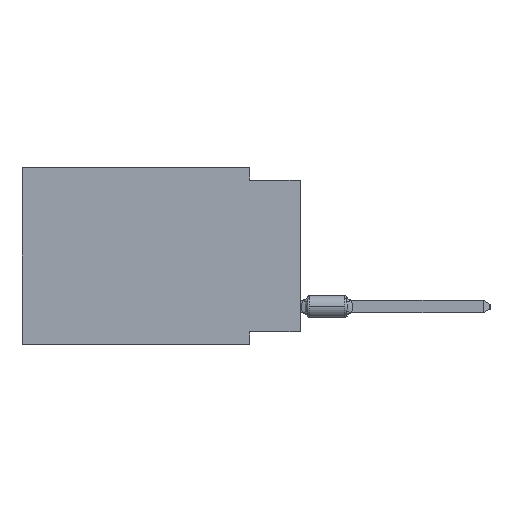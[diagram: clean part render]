
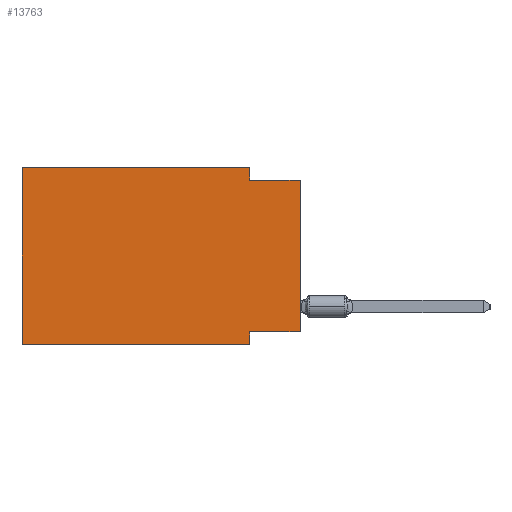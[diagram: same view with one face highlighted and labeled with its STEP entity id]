
A CAD part, left-side view. The second image highlights one B-rep face of the part: STEP entity #13763.
In plain terms, the highlighted planar face has unit normal (-1, 0, 0).
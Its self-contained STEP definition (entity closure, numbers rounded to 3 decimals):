
#1804 = CARTESIAN_POINT ( 'NONE',  ( 0., 13.97, 0. ) ) ;
#2532 = VERTEX_POINT ( 'NONE', #74510 ) ;
#4743 = VERTEX_POINT ( 'NONE', #37701 ) ;
#6497 = CARTESIAN_POINT ( 'NONE',  ( 0., 2.54, -8.255 ) ) ;
#6792 = DIRECTION ( 'NONE',  ( 0., -1., 0. ) ) ;
#8839 = DIRECTION ( 'NONE',  ( 0., -1., 0. ) ) ;
#11385 = EDGE_CURVE ( 'NONE', #55687, #71116, #38033, .T. ) ;
#11676 = VERTEX_POINT ( 'NONE', #31573 ) ;
#13763 = ADVANCED_FACE ( 'NONE', ( #26421 ), #49687, .F. ) ;
#14637 = VERTEX_POINT ( 'NONE', #60135 ) ;
#14918 = VECTOR ( 'NONE', #97933, 1000. ) ;
#18485 = CARTESIAN_POINT ( 'NONE',  ( 0., 13.97, 0. ) ) ;
#21671 = VERTEX_POINT ( 'NONE', #64441 ) ;
#23043 = LINE ( 'NONE', #67661, #14918 ) ;
#23168 = DIRECTION ( 'NONE',  ( 0., 0., -1. ) ) ;
#23503 = EDGE_CURVE ( 'NONE', #11676, #72707, #46404, .T. ) ;
#25033 = EDGE_CURVE ( 'NONE', #2532, #4743, #72565, .T. ) ;
#25195 = ORIENTED_EDGE ( 'NONE', *, *, #33677, .F. ) ;
#26421 = FACE_OUTER_BOUND ( 'NONE', #36761, .T. ) ;
#28302 = LINE ( 'NONE', #72433, #88564 ) ;
#31462 = ORIENTED_EDGE ( 'NONE', *, *, #58525, .T. ) ;
#31573 = CARTESIAN_POINT ( 'NONE',  ( 0., 13.97, 0. ) ) ;
#32923 = CARTESIAN_POINT ( 'NONE',  ( 0., 2.54, 0. ) ) ;
#33677 = EDGE_CURVE ( 'NONE', #2532, #55687, #85580, .T. ) ;
#34881 = CARTESIAN_POINT ( 'NONE',  ( 0., 0., 0. ) ) ;
#35316 = VECTOR ( 'NONE', #8839, 1000. ) ;
#36761 = EDGE_LOOP ( 'NONE', ( #65726, #79341, #88695, #41415, #40540, #31462, #63442, #25195 ) ) ;
#37701 = CARTESIAN_POINT ( 'NONE',  ( 0., 0., -0.635 ) ) ;
#38033 = LINE ( 'NONE', #60830, #38064 ) ;
#38064 = VECTOR ( 'NONE', #23168, 1000. ) ;
#40540 = ORIENTED_EDGE ( 'NONE', *, *, #73470, .F. ) ;
#40972 = VECTOR ( 'NONE', #6792, 1000. ) ;
#41415 = ORIENTED_EDGE ( 'NONE', *, *, #23503, .F. ) ;
#46404 = LINE ( 'NONE', #53337, #40972 ) ;
#46496 = CARTESIAN_POINT ( 'NONE',  ( 0., 13.97, -8.89 ) ) ;
#48286 = DIRECTION ( 'NONE',  ( 0., 0., 1. ) ) ;
#49687 = PLANE ( 'NONE',  #96887 ) ;
#52313 = EDGE_CURVE ( 'NONE', #72707, #14637, #28302, .T. ) ;
#53337 = CARTESIAN_POINT ( 'NONE',  ( 0., 13.97, 0. ) ) ;
#54364 = DIRECTION ( 'NONE',  ( 0., 0., 1. ) ) ;
#54808 = DIRECTION ( 'NONE',  ( 0., 1., 0. ) ) ;
#55396 = LINE ( 'NONE', #46496, #35316 ) ;
#55687 = VERTEX_POINT ( 'NONE', #6497 ) ;
#56162 = DIRECTION ( 'NONE',  ( 0., 0., -1. ) ) ;
#58525 = EDGE_CURVE ( 'NONE', #21671, #71116, #55396, .T. ) ;
#60135 = CARTESIAN_POINT ( 'NONE',  ( 0., 2.54, -0.635 ) ) ;
#60830 = CARTESIAN_POINT ( 'NONE',  ( 0., 2.54, -8.89 ) ) ;
#61460 = EDGE_CURVE ( 'NONE', #14637, #4743, #23043, .T. ) ;
#63442 = ORIENTED_EDGE ( 'NONE', *, *, #11385, .F. ) ;
#64441 = CARTESIAN_POINT ( 'NONE',  ( 0., 13.97, -8.89 ) ) ;
#64725 = VECTOR ( 'NONE', #54364, 1000. ) ;
#64823 = VECTOR ( 'NONE', #54808, 1000. ) ;
#65726 = ORIENTED_EDGE ( 'NONE', *, *, #25033, .T. ) ;
#67661 = CARTESIAN_POINT ( 'NONE',  ( 0., 0., -0.635 ) ) ;
#71116 = VERTEX_POINT ( 'NONE', #94997 ) ;
#72433 = CARTESIAN_POINT ( 'NONE',  ( 0., 2.54, 0. ) ) ;
#72565 = LINE ( 'NONE', #34881, #81069 ) ;
#72707 = VERTEX_POINT ( 'NONE', #32923 ) ;
#73470 = EDGE_CURVE ( 'NONE', #21671, #11676, #77192, .T. ) ;
#74510 = CARTESIAN_POINT ( 'NONE',  ( 0., 0., -8.255 ) ) ;
#77192 = LINE ( 'NONE', #1804, #64725 ) ;
#79341 = ORIENTED_EDGE ( 'NONE', *, *, #61460, .F. ) ;
#79387 = DIRECTION ( 'NONE',  ( 0., 0., -1. ) ) ;
#81069 = VECTOR ( 'NONE', #48286, 1000. ) ;
#85580 = LINE ( 'NONE', #93025, #64823 ) ;
#88564 = VECTOR ( 'NONE', #79387, 1000. ) ;
#88695 = ORIENTED_EDGE ( 'NONE', *, *, #52313, .F. ) ;
#93025 = CARTESIAN_POINT ( 'NONE',  ( 0., 0., -8.255 ) ) ;
#93873 = DIRECTION ( 'NONE',  ( 1., 0., 0. ) ) ;
#94997 = CARTESIAN_POINT ( 'NONE',  ( 0., 2.54, -8.89 ) ) ;
#96887 = AXIS2_PLACEMENT_3D ( 'NONE', #18485, #93873, #56162 ) ;
#97933 = DIRECTION ( 'NONE',  ( 0., -1., 0. ) ) ;
